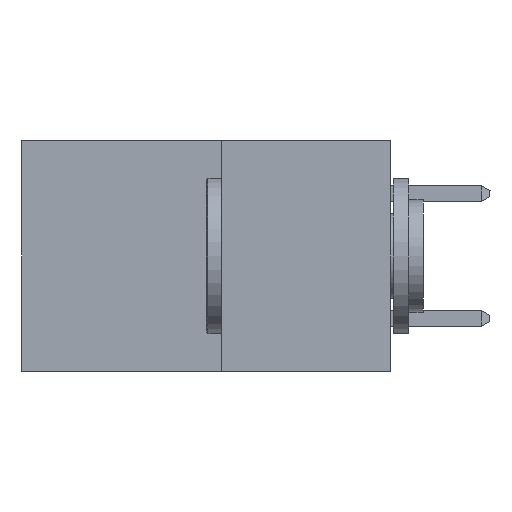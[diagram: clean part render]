
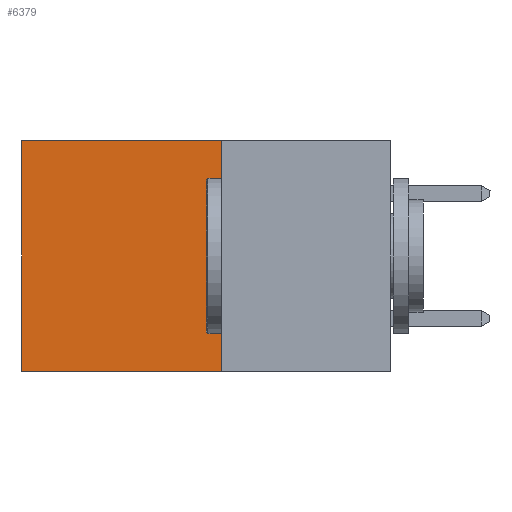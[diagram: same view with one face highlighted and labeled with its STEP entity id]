
A CAD part, left-side view. The second image highlights one B-rep face of the part: STEP entity #6379.
In plain terms, the highlighted planar face has unit normal (-1, 0, 0).
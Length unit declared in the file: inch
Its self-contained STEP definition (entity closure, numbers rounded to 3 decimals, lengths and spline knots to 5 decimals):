
#214 = CARTESIAN_POINT ( 'NONE',  ( 0.277, 0.27, 0. ) ) ;
#791 = DIRECTION ( 'NONE',  ( 0., 0., -1. ) ) ;
#1186 = VECTOR ( 'NONE', #2503, 39.37008 ) ;
#1323 = LINE ( 'NONE', #1778, #4044 ) ;
#1344 = CARTESIAN_POINT ( 'NONE',  ( 0.277, 0.59, -0.37 ) ) ;
#1452 = EDGE_CURVE ( 'NONE', #8376, #5644, #10044, .T. ) ;
#1560 = LINE ( 'NONE', #1344, #1186 ) ;
#1705 = DIRECTION ( 'NONE',  ( 0., 1., 0. ) ) ;
#1778 = CARTESIAN_POINT ( 'NONE',  ( 0.277, 0.27, -0.37 ) ) ;
#2122 = EDGE_CURVE ( 'NONE', #5644, #12698, #1323, .T. ) ;
#2392 = CARTESIAN_POINT ( 'NONE',  ( 0.277, 0.27, -0.37 ) ) ;
#2503 = DIRECTION ( 'NONE',  ( 0., 0., -1. ) ) ;
#2666 = LINE ( 'NONE', #214, #8020 ) ;
#2775 = PLANE ( 'NONE',  #7722 ) ;
#3162 = ORIENTED_EDGE ( 'NONE', *, *, #4625, .T. ) ;
#3736 = FACE_OUTER_BOUND ( 'NONE', #4846, .T. ) ;
#3944 = CARTESIAN_POINT ( 'NONE',  ( 0.277, 0.27, -0.37 ) ) ;
#4044 = VECTOR ( 'NONE', #13328, 39.37008 ) ;
#4577 = CARTESIAN_POINT ( 'NONE',  ( 0.277, 0.27, -0.37 ) ) ;
#4625 = EDGE_CURVE ( 'NONE', #8376, #10390, #2666, .T. ) ;
#4781 = ORIENTED_EDGE ( 'NONE', *, *, #2122, .F. ) ;
#4846 = EDGE_LOOP ( 'NONE', ( #7780, #4781, #11746, #3162 ) ) ;
#5051 = DIRECTION ( 'NONE',  ( 1., 0., 0. ) ) ;
#5644 = VERTEX_POINT ( 'NONE', #4577 ) ;
#6379 = ADVANCED_FACE ( 'NONE', ( #3736 ), #2775, .F. ) ;
#7307 = VECTOR ( 'NONE', #791, 39.37008 ) ;
#7644 = CARTESIAN_POINT ( 'NONE',  ( 0.277, 0.59, 0. ) ) ;
#7722 = AXIS2_PLACEMENT_3D ( 'NONE', #3944, #5051, #12142 ) ;
#7780 = ORIENTED_EDGE ( 'NONE', *, *, #11286, .T. ) ;
#8020 = VECTOR ( 'NONE', #1705, 39.37008 ) ;
#8376 = VERTEX_POINT ( 'NONE', #9187 ) ;
#9187 = CARTESIAN_POINT ( 'NONE',  ( 0.277, 0.27, 0. ) ) ;
#10044 = LINE ( 'NONE', #2392, #7307 ) ;
#10390 = VERTEX_POINT ( 'NONE', #7644 ) ;
#11286 = EDGE_CURVE ( 'NONE', #10390, #12698, #1560, .T. ) ;
#11746 = ORIENTED_EDGE ( 'NONE', *, *, #1452, .F. ) ;
#12142 = DIRECTION ( 'NONE',  ( 0., 0., -1. ) ) ;
#12698 = VERTEX_POINT ( 'NONE', #13580 ) ;
#13328 = DIRECTION ( 'NONE',  ( 0., 1., 0. ) ) ;
#13580 = CARTESIAN_POINT ( 'NONE',  ( 0.277, 0.59, -0.37 ) ) ;
